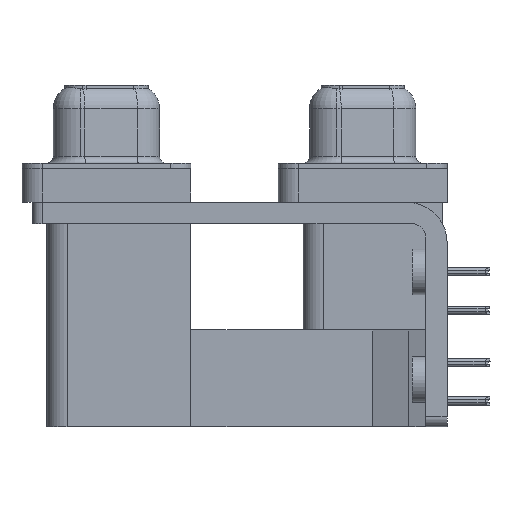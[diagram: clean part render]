
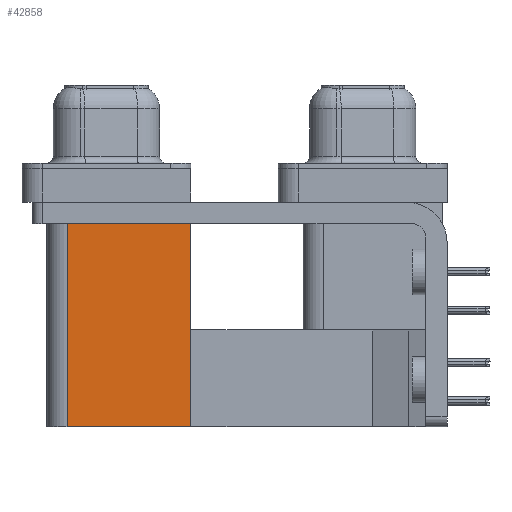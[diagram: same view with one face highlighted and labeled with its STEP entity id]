
A CAD part, left-side view. The second image highlights one B-rep face of the part: STEP entity #42858.
In plain terms, the highlighted planar face has unit normal (-1, 0, 0).
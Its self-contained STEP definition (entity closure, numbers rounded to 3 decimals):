
#3429 = VERTEX_POINT ( 'NONE', #33487 ) ;
#3786 = EDGE_CURVE ( 'NONE', #12919, #40117, #35721, .T. ) ;
#4289 = ORIENTED_EDGE ( 'NONE', *, *, #22403, .T. ) ;
#4871 = DIRECTION ( 'NONE',  ( 0., 1., 0. ) ) ;
#5072 = CARTESIAN_POINT ( 'NONE',  ( 3.79, 12.775, -19.2 ) ) ;
#7327 = VECTOR ( 'NONE', #8224, 1000. ) ;
#8224 = DIRECTION ( 'NONE',  ( 0., 0., 1. ) ) ;
#10484 = CARTESIAN_POINT ( 'NONE',  ( 3.79, 12.775, -2.5 ) ) ;
#11843 = LINE ( 'NONE', #25587, #42436 ) ;
#12685 = CARTESIAN_POINT ( 'NONE',  ( 3.79, 21.975, -19.2 ) ) ;
#12919 = VERTEX_POINT ( 'NONE', #12685 ) ;
#14485 = VECTOR ( 'NONE', #29977, 1000. ) ;
#15668 = CARTESIAN_POINT ( 'NONE',  ( 3.79, 12.775, -19.2 ) ) ;
#16749 = ORIENTED_EDGE ( 'NONE', *, *, #3786, .F. ) ;
#19481 = EDGE_CURVE ( 'NONE', #3429, #12919, #11843, .T. ) ;
#21986 = DIRECTION ( 'NONE',  ( 1., 0., 0. ) ) ;
#22403 = EDGE_CURVE ( 'NONE', #3429, #25195, #32960, .T. ) ;
#23950 = EDGE_CURVE ( 'NONE', #25195, #40117, #42401, .T. ) ;
#25195 = VERTEX_POINT ( 'NONE', #10484 ) ;
#25587 = CARTESIAN_POINT ( 'NONE',  ( 3.79, 12.775, -19.2 ) ) ;
#26707 = CARTESIAN_POINT ( 'NONE',  ( 3.79, 21.975, -2.5 ) ) ;
#28755 = DIRECTION ( 'NONE',  ( 0., 0., 1. ) ) ;
#29977 = DIRECTION ( 'NONE',  ( 0., 1., 0. ) ) ;
#32280 = ORIENTED_EDGE ( 'NONE', *, *, #23950, .T. ) ;
#32450 = VECTOR ( 'NONE', #28755, 1000. ) ;
#32567 = CARTESIAN_POINT ( 'NONE',  ( 3.79, 21.975, -19.2 ) ) ;
#32960 = LINE ( 'NONE', #5072, #7327 ) ;
#33349 = CARTESIAN_POINT ( 'NONE',  ( 3.79, 12.775, -2.5 ) ) ;
#33487 = CARTESIAN_POINT ( 'NONE',  ( 3.79, 12.775, -19.2 ) ) ;
#35721 = LINE ( 'NONE', #32567, #32450 ) ;
#35960 = AXIS2_PLACEMENT_3D ( 'NONE', #15668, #21986, #4871 ) ;
#36637 = EDGE_LOOP ( 'NONE', ( #32280, #16749, #42636, #4289 ) ) ;
#39316 = DIRECTION ( 'NONE',  ( 0., 1., 0. ) ) ;
#40117 = VERTEX_POINT ( 'NONE', #26707 ) ;
#42255 = PLANE ( 'NONE',  #35960 ) ;
#42401 = LINE ( 'NONE', #33349, #14485 ) ;
#42436 = VECTOR ( 'NONE', #39316, 1000. ) ;
#42636 = ORIENTED_EDGE ( 'NONE', *, *, #19481, .F. ) ;
#42858 = ADVANCED_FACE ( 'NONE', ( #42905 ), #42255, .F. ) ;
#42905 = FACE_OUTER_BOUND ( 'NONE', #36637, .T. ) ;
